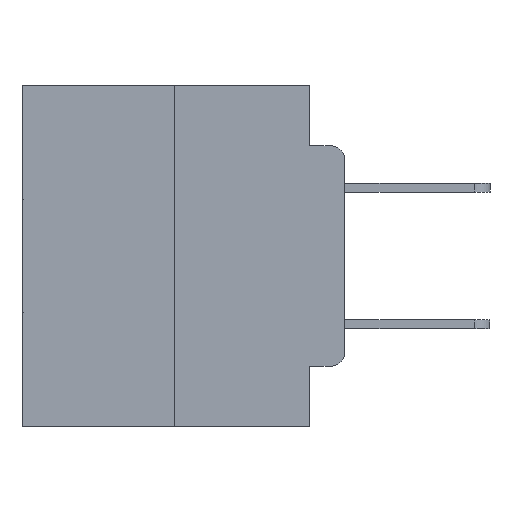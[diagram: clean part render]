
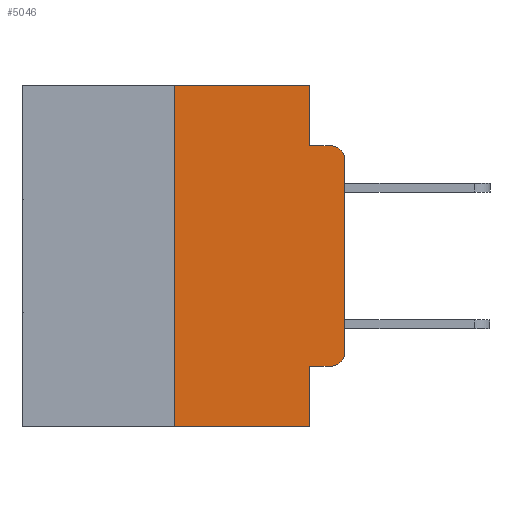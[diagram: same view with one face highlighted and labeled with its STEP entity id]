
A CAD part, left-side view. The second image highlights one B-rep face of the part: STEP entity #5046.
In plain terms, the highlighted planar face has unit normal (-1, 0, 0).
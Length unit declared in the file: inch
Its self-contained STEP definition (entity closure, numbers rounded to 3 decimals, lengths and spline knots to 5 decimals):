
#236 = LINE ( 'NONE', #21984, #16209 ) ;
#827 = EDGE_CURVE ( 'NONE', #23457, #15655, #6948, .T. ) ;
#1467 = ORIENTED_EDGE ( 'NONE', *, *, #9825, .F. ) ;
#2496 = CARTESIAN_POINT ( 'NONE',  ( 0., 0.051, 0. ) ) ;
#2682 = CARTESIAN_POINT ( 'NONE',  ( 0., 0.25, -0.5 ) ) ;
#2843 = ORIENTED_EDGE ( 'NONE', *, *, #827, .F. ) ;
#3076 = CARTESIAN_POINT ( 'NONE',  ( 0., 0.051, -0.0885 ) ) ;
#3706 = CIRCLE ( 'NONE', #22093, 0.02 ) ;
#3728 = EDGE_CURVE ( 'NONE', #16005, #17082, #15177, .T. ) ;
#3988 = CARTESIAN_POINT ( 'NONE',  ( 0., 0.02, -0.4115 ) ) ;
#5046 = ADVANCED_FACE ( 'NONE', ( #26763 ), #9922, .F. ) ;
#5477 = DIRECTION ( 'NONE',  ( 0., -1., 0. ) ) ;
#5795 = ORIENTED_EDGE ( 'NONE', *, *, #7894, .F. ) ;
#6423 = ORIENTED_EDGE ( 'NONE', *, *, #3728, .F. ) ;
#6679 = CARTESIAN_POINT ( 'NONE',  ( 0., 0.051, -0.5 ) ) ;
#6769 = ORIENTED_EDGE ( 'NONE', *, *, #22282, .T. ) ;
#6948 = LINE ( 'NONE', #7872, #11774 ) ;
#7872 = CARTESIAN_POINT ( 'NONE',  ( 0., 0.25, 0. ) ) ;
#7894 = EDGE_CURVE ( 'NONE', #17082, #20910, #26376, .T. ) ;
#8204 = VECTOR ( 'NONE', #19354, 39.37008 ) ;
#8397 = VECTOR ( 'NONE', #22712, 39.37008 ) ;
#8816 = CARTESIAN_POINT ( 'NONE',  ( 0., 0.02, -0.1085 ) ) ;
#9089 = CARTESIAN_POINT ( 'NONE',  ( 0., 0.02, -0.0885 ) ) ;
#9573 = DIRECTION ( 'NONE',  ( 0., -1., 0. ) ) ;
#9693 = CARTESIAN_POINT ( 'NONE',  ( 0., 0.25, 0. ) ) ;
#9825 = EDGE_CURVE ( 'NONE', #15655, #16005, #12011, .T. ) ;
#9878 = VECTOR ( 'NONE', #11394, 39.37008 ) ;
#9922 = PLANE ( 'NONE',  #25419 ) ;
#10830 = VERTEX_POINT ( 'NONE', #3988 ) ;
#10905 = DIRECTION ( 'NONE',  ( 0., 0., -1. ) ) ;
#10973 = ORIENTED_EDGE ( 'NONE', *, *, #23673, .T. ) ;
#11102 = DIRECTION ( 'NONE',  ( -1., 0., 0. ) ) ;
#11394 = DIRECTION ( 'NONE',  ( 0., -1., 0. ) ) ;
#11774 = VECTOR ( 'NONE', #20392, 39.37008 ) ;
#11895 = CARTESIAN_POINT ( 'NONE',  ( 0., 0.473, 0. ) ) ;
#11980 = DIRECTION ( 'NONE',  ( 1., 0., 0. ) ) ;
#12011 = LINE ( 'NONE', #22007, #23049 ) ;
#13394 = DIRECTION ( 'NONE',  ( 0., 0., -1. ) ) ;
#13397 = EDGE_CURVE ( 'NONE', #18305, #20910, #3706, .T. ) ;
#13831 = EDGE_LOOP ( 'NONE', ( #20985, #21635, #5795, #6423, #1467, #2843, #15145, #26176, #10973, #6769 ) ) ;
#14097 = EDGE_CURVE ( 'NONE', #23457, #22192, #14313, .T. ) ;
#14178 = VERTEX_POINT ( 'NONE', #21701 ) ;
#14313 = LINE ( 'NONE', #21442, #8204 ) ;
#15145 = ORIENTED_EDGE ( 'NONE', *, *, #14097, .T. ) ;
#15177 = LINE ( 'NONE', #22828, #8397 ) ;
#15585 = VECTOR ( 'NONE', #13394, 39.37008 ) ;
#15655 = VERTEX_POINT ( 'NONE', #9693 ) ;
#15805 = AXIS2_PLACEMENT_3D ( 'NONE', #23507, #11102, #25576 ) ;
#16005 = VERTEX_POINT ( 'NONE', #2496 ) ;
#16190 = EDGE_CURVE ( 'NONE', #21184, #18305, #26516, .T. ) ;
#16209 = VECTOR ( 'NONE', #9573, 39.37008 ) ;
#17082 = VERTEX_POINT ( 'NONE', #18575 ) ;
#18236 = CIRCLE ( 'NONE', #15805, 0.02 ) ;
#18305 = VERTEX_POINT ( 'NONE', #24954 ) ;
#18575 = CARTESIAN_POINT ( 'NONE',  ( 0., 0.051, -0.0885 ) ) ;
#19354 = DIRECTION ( 'NONE',  ( 0., -1., 0. ) ) ;
#20392 = DIRECTION ( 'NONE',  ( 0., 0., 1. ) ) ;
#20641 = CARTESIAN_POINT ( 'NONE',  ( 0., 0., -0.3915 ) ) ;
#20910 = VERTEX_POINT ( 'NONE', #9089 ) ;
#20985 = ORIENTED_EDGE ( 'NONE', *, *, #16190, .T. ) ;
#21023 = VECTOR ( 'NONE', #22084, 39.37008 ) ;
#21184 = VERTEX_POINT ( 'NONE', #20641 ) ;
#21442 = CARTESIAN_POINT ( 'NONE',  ( 0., 0.473, -0.5 ) ) ;
#21635 = ORIENTED_EDGE ( 'NONE', *, *, #13397, .T. ) ;
#21701 = CARTESIAN_POINT ( 'NONE',  ( 0., 0.051, -0.4115 ) ) ;
#21984 = CARTESIAN_POINT ( 'NONE',  ( 0., 0.051, -0.4115 ) ) ;
#22007 = CARTESIAN_POINT ( 'NONE',  ( 0., 0.473, 0. ) ) ;
#22084 = DIRECTION ( 'NONE',  ( 0., 0., 1. ) ) ;
#22093 = AXIS2_PLACEMENT_3D ( 'NONE', #8816, #23303, #10905 ) ;
#22192 = VERTEX_POINT ( 'NONE', #6679 ) ;
#22282 = EDGE_CURVE ( 'NONE', #10830, #21184, #18236, .T. ) ;
#22712 = DIRECTION ( 'NONE',  ( 0., 0., -1. ) ) ;
#22828 = CARTESIAN_POINT ( 'NONE',  ( 0., 0.051, 0. ) ) ;
#23049 = VECTOR ( 'NONE', #5477, 39.37008 ) ;
#23303 = DIRECTION ( 'NONE',  ( -1., 0., 0. ) ) ;
#23457 = VERTEX_POINT ( 'NONE', #2682 ) ;
#23507 = CARTESIAN_POINT ( 'NONE',  ( 0., 0.02, -0.3915 ) ) ;
#23671 = CARTESIAN_POINT ( 'NONE',  ( 0., 0.051, 0. ) ) ;
#23673 = EDGE_CURVE ( 'NONE', #14178, #10830, #236, .T. ) ;
#24049 = CARTESIAN_POINT ( 'NONE',  ( 0., 0., 0. ) ) ;
#24954 = CARTESIAN_POINT ( 'NONE',  ( 0., 0., -0.1085 ) ) ;
#25043 = EDGE_CURVE ( 'NONE', #14178, #22192, #26595, .T. ) ;
#25419 = AXIS2_PLACEMENT_3D ( 'NONE', #11895, #11980, #26466 ) ;
#25576 = DIRECTION ( 'NONE',  ( 0., 0., -1. ) ) ;
#26176 = ORIENTED_EDGE ( 'NONE', *, *, #25043, .F. ) ;
#26376 = LINE ( 'NONE', #3076, #9878 ) ;
#26466 = DIRECTION ( 'NONE',  ( 0., 0., -1. ) ) ;
#26516 = LINE ( 'NONE', #24049, #21023 ) ;
#26595 = LINE ( 'NONE', #23671, #15585 ) ;
#26763 = FACE_OUTER_BOUND ( 'NONE', #13831, .T. ) ;
